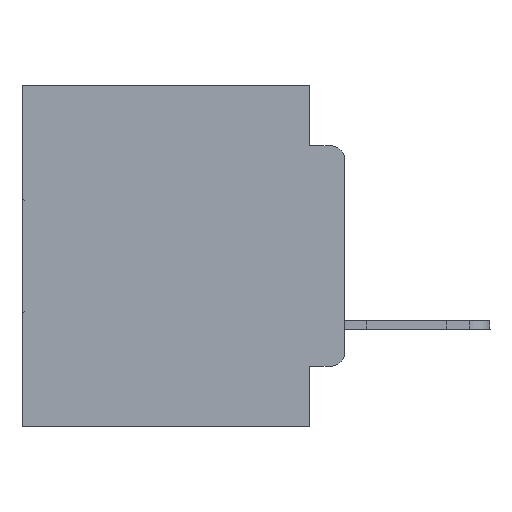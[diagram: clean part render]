
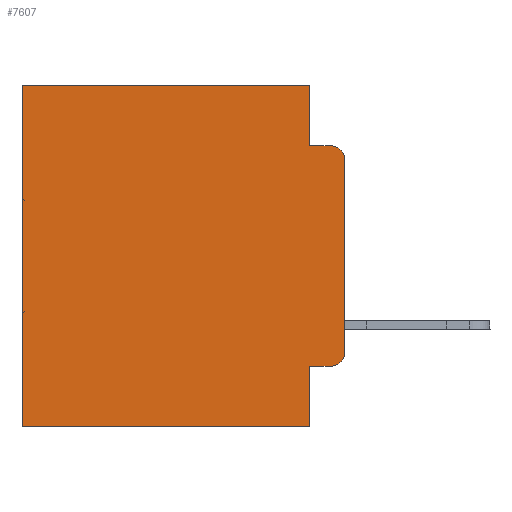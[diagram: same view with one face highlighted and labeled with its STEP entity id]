
A CAD part, left-side view. The second image highlights one B-rep face of the part: STEP entity #7607.
In plain terms, the highlighted planar face has unit normal (-1, 0, 0).
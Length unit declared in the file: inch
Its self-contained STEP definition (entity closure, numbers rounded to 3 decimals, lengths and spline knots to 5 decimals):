
#299 = LINE ( 'NONE', #10508, #12406 ) ;
#415 = CARTESIAN_POINT ( 'NONE',  ( 0.298, 0.473, 0. ) ) ;
#641 = EDGE_CURVE ( 'NONE', #14794, #21291, #10964, .T. ) ;
#694 = ORIENTED_EDGE ( 'NONE', *, *, #641, .F. ) ;
#825 = LINE ( 'NONE', #415, #26204 ) ;
#1004 = VECTOR ( 'NONE', #8552, 39.37008 ) ;
#2372 = EDGE_CURVE ( 'NONE', #22522, #13032, #8213, .T. ) ;
#2723 = DIRECTION ( 'NONE',  ( 0., 1., 0. ) ) ;
#3295 = AXIS2_PLACEMENT_3D ( 'NONE', #15126, #10448, #27617 ) ;
#4123 = LINE ( 'NONE', #19792, #19643 ) ;
#4383 = DIRECTION ( 'NONE',  ( 0., 0., -1. ) ) ;
#4696 = PLANE ( 'NONE',  #23252 ) ;
#5256 = LINE ( 'NONE', #12857, #27570 ) ;
#6546 = CARTESIAN_POINT ( 'NONE',  ( 0.298, 0., -0.3915 ) ) ;
#6774 = CARTESIAN_POINT ( 'NONE',  ( 0.298, 0.051, 0. ) ) ;
#7014 = CARTESIAN_POINT ( 'NONE',  ( 0.298, 0., 0. ) ) ;
#7198 = ORIENTED_EDGE ( 'NONE', *, *, #8110, .F. ) ;
#7607 = ADVANCED_FACE ( 'NONE', ( #30721 ), #4696, .F. ) ;
#7651 = VERTEX_POINT ( 'NONE', #21637 ) ;
#7951 = CARTESIAN_POINT ( 'NONE',  ( 0.298, 0.02, -0.0885 ) ) ;
#8110 = EDGE_CURVE ( 'NONE', #30272, #14794, #19358, .T. ) ;
#8213 = CIRCLE ( 'NONE', #14205, 0.02 ) ;
#8512 = VERTEX_POINT ( 'NONE', #27808 ) ;
#8552 = DIRECTION ( 'NONE',  ( 0., 0., -1. ) ) ;
#8582 = CARTESIAN_POINT ( 'NONE',  ( 0.298, 0.02, -0.4115 ) ) ;
#8704 = CARTESIAN_POINT ( 'NONE',  ( 0.298, 0.051, -0.4115 ) ) ;
#8712 = VECTOR ( 'NONE', #8958, 39.37008 ) ;
#8958 = DIRECTION ( 'NONE',  ( 0., 0., -1. ) ) ;
#9088 = EDGE_CURVE ( 'NONE', #30272, #8512, #5256, .T. ) ;
#9379 = VECTOR ( 'NONE', #12489, 39.37008 ) ;
#9611 = CARTESIAN_POINT ( 'NONE',  ( 0.298, 0.051, -0.5 ) ) ;
#9921 = DIRECTION ( 'NONE',  ( -1., 0., 0. ) ) ;
#10448 = DIRECTION ( 'NONE',  ( -1., 0., 0. ) ) ;
#10508 = CARTESIAN_POINT ( 'NONE',  ( 0.298, 0.051, 0. ) ) ;
#10913 = LINE ( 'NONE', #29202, #9379 ) ;
#10964 = LINE ( 'NONE', #25939, #29893 ) ;
#11029 = DIRECTION ( 'NONE',  ( 0., -1., 0. ) ) ;
#12267 = EDGE_CURVE ( 'NONE', #15052, #22522, #10913, .T. ) ;
#12406 = VECTOR ( 'NONE', #22727, 39.37008 ) ;
#12489 = DIRECTION ( 'NONE',  ( 0., -1., 0. ) ) ;
#12647 = ORIENTED_EDGE ( 'NONE', *, *, #12267, .T. ) ;
#12857 = CARTESIAN_POINT ( 'NONE',  ( 0.298, 0., 0. ) ) ;
#13032 = VERTEX_POINT ( 'NONE', #6546 ) ;
#13780 = CARTESIAN_POINT ( 'NONE',  ( 0.298, 0.051, 0. ) ) ;
#13966 = VERTEX_POINT ( 'NONE', #9611 ) ;
#14205 = AXIS2_PLACEMENT_3D ( 'NONE', #24773, #9921, #15125 ) ;
#14267 = EDGE_CURVE ( 'NONE', #7651, #13032, #30174, .T. ) ;
#14794 = VERTEX_POINT ( 'NONE', #15303 ) ;
#14803 = DIRECTION ( 'NONE',  ( 0., 0., -1. ) ) ;
#14964 = ORIENTED_EDGE ( 'NONE', *, *, #14267, .F. ) ;
#15052 = VERTEX_POINT ( 'NONE', #8704 ) ;
#15125 = DIRECTION ( 'NONE',  ( 0., 0., -1. ) ) ;
#15126 = CARTESIAN_POINT ( 'NONE',  ( 0.298, 0.02, -0.1085 ) ) ;
#15303 = CARTESIAN_POINT ( 'NONE',  ( 0.298, 0.051, -0.0885 ) ) ;
#15771 = ORIENTED_EDGE ( 'NONE', *, *, #24900, .T. ) ;
#16521 = ORIENTED_EDGE ( 'NONE', *, *, #23599, .F. ) ;
#18462 = ORIENTED_EDGE ( 'NONE', *, *, #9088, .T. ) ;
#19358 = LINE ( 'NONE', #6774, #8712 ) ;
#19643 = VECTOR ( 'NONE', #2723, 39.37008 ) ;
#19682 = CARTESIAN_POINT ( 'NONE',  ( 0.298, 0.473, -0.5 ) ) ;
#19792 = CARTESIAN_POINT ( 'NONE',  ( 0.298, 0., -0.5 ) ) ;
#20613 = DIRECTION ( 'NONE',  ( 0., 1., 0. ) ) ;
#20615 = EDGE_CURVE ( 'NONE', #8512, #27633, #825, .T. ) ;
#20912 = ORIENTED_EDGE ( 'NONE', *, *, #20615, .T. ) ;
#21291 = VERTEX_POINT ( 'NONE', #7951 ) ;
#21637 = CARTESIAN_POINT ( 'NONE',  ( 0.298, 0., -0.1085 ) ) ;
#22522 = VERTEX_POINT ( 'NONE', #8582 ) ;
#22568 = CIRCLE ( 'NONE', #3295, 0.02 ) ;
#22612 = ORIENTED_EDGE ( 'NONE', *, *, #23459, .F. ) ;
#22727 = DIRECTION ( 'NONE',  ( 0., 0., -1. ) ) ;
#22981 = CARTESIAN_POINT ( 'NONE',  ( 0.298, 0., 0. ) ) ;
#23252 = AXIS2_PLACEMENT_3D ( 'NONE', #7014, #28894, #4383 ) ;
#23459 = EDGE_CURVE ( 'NONE', #13966, #27633, #4123, .T. ) ;
#23599 = EDGE_CURVE ( 'NONE', #15052, #13966, #299, .T. ) ;
#23769 = ORIENTED_EDGE ( 'NONE', *, *, #2372, .T. ) ;
#24773 = CARTESIAN_POINT ( 'NONE',  ( 0.298, 0.02, -0.3915 ) ) ;
#24900 = EDGE_CURVE ( 'NONE', #7651, #21291, #22568, .T. ) ;
#25939 = CARTESIAN_POINT ( 'NONE',  ( 0.298, 0.051, -0.0885 ) ) ;
#26204 = VECTOR ( 'NONE', #14803, 39.37008 ) ;
#27570 = VECTOR ( 'NONE', #20613, 39.37008 ) ;
#27617 = DIRECTION ( 'NONE',  ( 0., 0., -1. ) ) ;
#27633 = VERTEX_POINT ( 'NONE', #19682 ) ;
#27808 = CARTESIAN_POINT ( 'NONE',  ( 0.298, 0.473, 0. ) ) ;
#28894 = DIRECTION ( 'NONE',  ( 1., 0., 0. ) ) ;
#29202 = CARTESIAN_POINT ( 'NONE',  ( 0.298, 0.051, -0.4115 ) ) ;
#29893 = VECTOR ( 'NONE', #11029, 39.37008 ) ;
#30174 = LINE ( 'NONE', #22981, #1004 ) ;
#30272 = VERTEX_POINT ( 'NONE', #13780 ) ;
#30721 = FACE_OUTER_BOUND ( 'NONE', #31238, .T. ) ;
#31238 = EDGE_LOOP ( 'NONE', ( #14964, #15771, #694, #7198, #18462, #20912, #22612, #16521, #12647, #23769 ) ) ;
